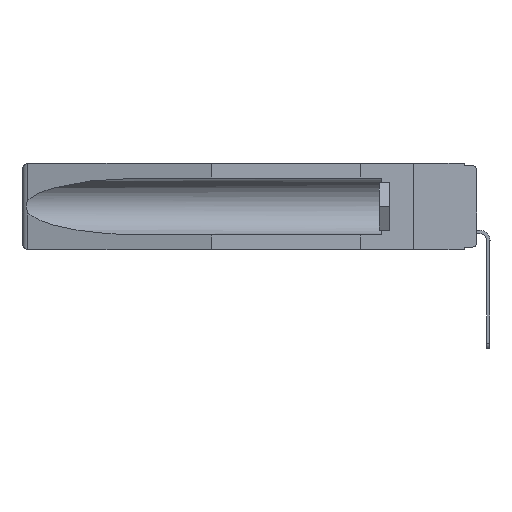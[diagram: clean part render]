
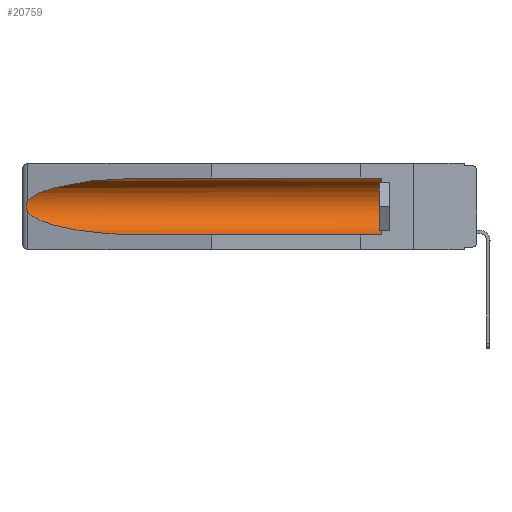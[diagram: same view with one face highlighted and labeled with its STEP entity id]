
A CAD part, left-side view. The second image highlights one B-rep face of the part: STEP entity #20759.
In plain terms, the highlighted cylindrical face has radius 2.857 mm (diameter 5.715 mm), a partial arc.
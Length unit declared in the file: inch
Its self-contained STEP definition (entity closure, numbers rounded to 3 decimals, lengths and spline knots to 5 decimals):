
#545 = CARTESIAN_POINT ( 'NONE',  ( 0.25451, 1.48313, -0.09465 ) ) ;
#551 = EDGE_CURVE ( 'NONE', #10197, #5527, #10877, .T. ) ;
#871 = LINE ( 'NONE', #19132, #9181 ) ;
#1275 = CARTESIAN_POINT ( 'NONE',  ( 0.155, 0.126, -0.1715 ) ) ;
#1717 = AXIS2_PLACEMENT_3D ( 'NONE', #1275, #20711, #12238 ) ;
#1752 = ORIENTED_EDGE ( 'NONE', *, *, #13686, .T. ) ;
#1841 = CARTESIAN_POINT ( 'NONE',  ( 0.155, 1.07973, -0.284 ) ) ;
#2256 =( BOUNDED_CURVE ( )  B_SPLINE_CURVE ( 3, ( #8428, #19797, #10121, #1841 ),
 .UNSPECIFIED., .F., .F. ) 
 B_SPLINE_CURVE_WITH_KNOTS ( ( 4, 4 ),
 ( 0.1948, 1.5708 ),
 .UNSPECIFIED. ) 
 CURVE ( )  GEOMETRIC_REPRESENTATION_ITEM ( )  RATIONAL_B_SPLINE_CURVE ( ( 1., 0.848, 0.848, 1. ) ) 
 REPRESENTATION_ITEM ( '' )  );
#2452 = CARTESIAN_POINT ( 'NONE',  ( 0.26597, 1.5296, -0.19026 ) ) ;
#2774 = CARTESIAN_POINT ( 'NONE',  ( 0.26654, 1.53092, -0.15636 ) ) ;
#3045 = FACE_OUTER_BOUND ( 'NONE', #13981, .T. ) ;
#3292 = CARTESIAN_POINT ( 'NONE',  ( 0.26537, 1.52718, -0.14972 ) ) ;
#3406 = ORIENTED_EDGE ( 'NONE', *, *, #8305, .T. ) ;
#3472 = DIRECTION ( 'NONE',  ( 0., 1., 0. ) ) ;
#3712 = CARTESIAN_POINT ( 'NONE',  ( 0.155, 0.126, -0.059 ) ) ;
#4481 = DIRECTION ( 'NONE',  ( 0., 1., 0. ) ) ;
#4880 = ORIENTED_EDGE ( 'NONE', *, *, #6738, .T. ) ;
#4967 = DIRECTION ( 'NONE',  ( 0., 0., 1. ) ) ;
#4996 =( BOUNDED_CURVE ( )  B_SPLINE_CURVE ( 3, ( #5113, #9769, #545, #3292 ),
 .UNSPECIFIED., .F., .F. ) 
 B_SPLINE_CURVE_WITH_KNOTS ( ( 4, 4 ),
 ( 4.71239, 6.08839 ),
 .UNSPECIFIED. ) 
 CURVE ( )  GEOMETRIC_REPRESENTATION_ITEM ( )  RATIONAL_B_SPLINE_CURVE ( ( 1., 0.848, 0.848, 1. ) ) 
 REPRESENTATION_ITEM ( '' )  );
#5113 = CARTESIAN_POINT ( 'NONE',  ( 0.155, 1.07973, -0.059 ) ) ;
#5527 = VERTEX_POINT ( 'NONE', #3712 ) ;
#5631 = CARTESIAN_POINT ( 'NONE',  ( 0.155, -0.30754, -0.284 ) ) ;
#5962 = CARTESIAN_POINT ( 'NONE',  ( 0.2675, 1.53308, -0.16763 ) ) ;
#6738 = EDGE_CURVE ( 'NONE', #13118, #20661, #4996, .T. ) ;
#6930 = EDGE_CURVE ( 'NONE', #10197, #16799, #12008, .T. ) ;
#6968 = CARTESIAN_POINT ( 'NONE',  ( 0.26597, 1.52961, -0.15275 ) ) ;
#7101 = B_SPLINE_CURVE_WITH_KNOTS ( 'NONE', 3,
 ( #17021, #6968, #2774, #12241, #5962, #8928, #10527, #19920, #2452, #15642 ),
 .UNSPECIFIED., .F., .F.,
 ( 4, 2, 2, 2, 4 ),
 ( 0., 0.00029, 0.00058, 0.00087, 0.00117 ),
 .UNSPECIFIED. ) ;
#8305 = EDGE_CURVE ( 'NONE', #5527, #13118, #871, .T. ) ;
#8428 = CARTESIAN_POINT ( 'NONE',  ( 0.26537, 1.52718, -0.19328 ) ) ;
#8928 = CARTESIAN_POINT ( 'NONE',  ( 0.2675, 1.53308, -0.17534 ) ) ;
#9012 = DIRECTION ( 'NONE',  ( 0., 1., 0. ) ) ;
#9181 = VECTOR ( 'NONE', #4481, 39.37008 ) ;
#9769 = CARTESIAN_POINT ( 'NONE',  ( 0.21114, 1.30732, -0.059 ) ) ;
#9985 = CARTESIAN_POINT ( 'NONE',  ( 0.155, 1.07973, -0.284 ) ) ;
#10121 = CARTESIAN_POINT ( 'NONE',  ( 0.21114, 1.30732, -0.284 ) ) ;
#10197 = VERTEX_POINT ( 'NONE', #18869 ) ;
#10527 = CARTESIAN_POINT ( 'NONE',  ( 0.2673, 1.53269, -0.17917 ) ) ;
#10877 = CIRCLE ( 'NONE', #1717, 0.1125 ) ;
#11277 = ORIENTED_EDGE ( 'NONE', *, *, #12140, .T. ) ;
#11654 = CARTESIAN_POINT ( 'NONE',  ( 0.26537, 1.52718, -0.19328 ) ) ;
#11875 = CARTESIAN_POINT ( 'NONE',  ( 0.155, 1.07973, -0.059 ) ) ;
#12008 = LINE ( 'NONE', #5631, #15598 ) ;
#12140 = EDGE_CURVE ( 'NONE', #16138, #16799, #2256, .T. ) ;
#12238 = DIRECTION ( 'NONE',  ( 0., 0., 1. ) ) ;
#12241 = CARTESIAN_POINT ( 'NONE',  ( 0.2673, 1.5327, -0.16383 ) ) ;
#12628 = CARTESIAN_POINT ( 'NONE',  ( 0.26537, 1.52718, -0.14972 ) ) ;
#12827 = CYLINDRICAL_SURFACE ( 'NONE', #16898, 0.1125 ) ;
#13118 = VERTEX_POINT ( 'NONE', #11875 ) ;
#13686 = EDGE_CURVE ( 'NONE', #20661, #16138, #7101, .T. ) ;
#13981 = EDGE_LOOP ( 'NONE', ( #4880, #1752, #11277, #17800, #14422, #3406 ) ) ;
#14422 = ORIENTED_EDGE ( 'NONE', *, *, #551, .T. ) ;
#15598 = VECTOR ( 'NONE', #9012, 39.37008 ) ;
#15642 = CARTESIAN_POINT ( 'NONE',  ( 0.26537, 1.52718, -0.19328 ) ) ;
#16138 = VERTEX_POINT ( 'NONE', #11654 ) ;
#16799 = VERTEX_POINT ( 'NONE', #9985 ) ;
#16898 = AXIS2_PLACEMENT_3D ( 'NONE', #17712, #3472, #4967 ) ;
#17021 = CARTESIAN_POINT ( 'NONE',  ( 0.26537, 1.52718, -0.14972 ) ) ;
#17712 = CARTESIAN_POINT ( 'NONE',  ( 0.155, -0.30754, -0.1715 ) ) ;
#17800 = ORIENTED_EDGE ( 'NONE', *, *, #6930, .F. ) ;
#18869 = CARTESIAN_POINT ( 'NONE',  ( 0.155, 0.126, -0.284 ) ) ;
#19132 = CARTESIAN_POINT ( 'NONE',  ( 0.155, -0.30754, -0.059 ) ) ;
#19797 = CARTESIAN_POINT ( 'NONE',  ( 0.25451, 1.48313, -0.24835 ) ) ;
#19920 = CARTESIAN_POINT ( 'NONE',  ( 0.26655, 1.53094, -0.18657 ) ) ;
#20661 = VERTEX_POINT ( 'NONE', #12628 ) ;
#20711 = DIRECTION ( 'NONE',  ( 0., -1., 0. ) ) ;
#20759 = ADVANCED_FACE ( 'NONE', ( #3045 ), #12827, .F. ) ;
